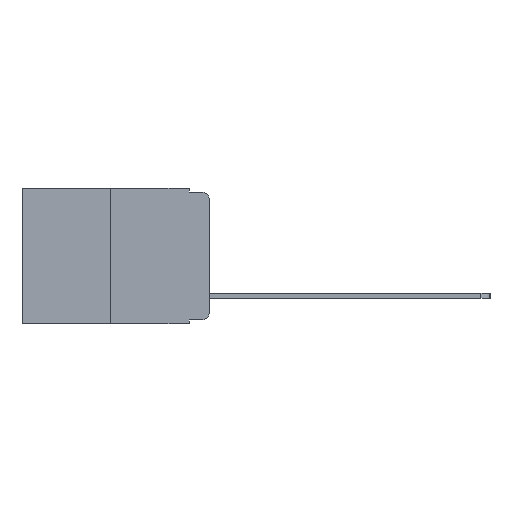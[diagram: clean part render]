
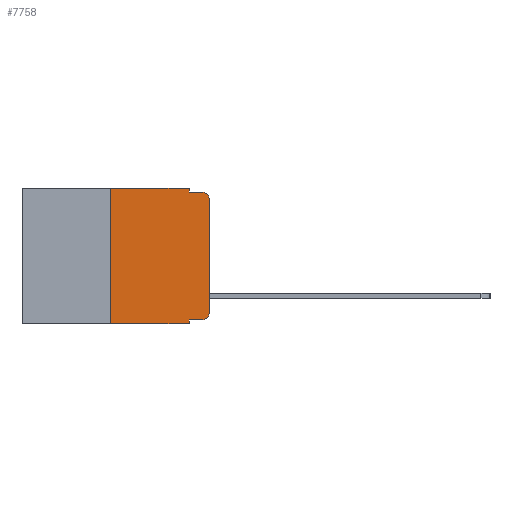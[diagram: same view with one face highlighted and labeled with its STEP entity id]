
A CAD part, left-side view. The second image highlights one B-rep face of the part: STEP entity #7758.
In plain terms, the highlighted planar face has unit normal (-1, 0, 0).
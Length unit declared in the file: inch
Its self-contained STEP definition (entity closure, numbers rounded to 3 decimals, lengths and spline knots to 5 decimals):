
#94 = CARTESIAN_POINT ( 'NONE',  ( 0., 0.051, 0. ) ) ;
#453 = VERTEX_POINT ( 'NONE', #15415 ) ;
#502 = VERTEX_POINT ( 'NONE', #5498 ) ;
#616 = VECTOR ( 'NONE', #14055, 39.37008 ) ;
#1423 = CARTESIAN_POINT ( 'NONE',  ( 0., 0.473, 0. ) ) ;
#1631 = DIRECTION ( 'NONE',  ( 0., -1., 0. ) ) ;
#1732 = LINE ( 'NONE', #10804, #14436 ) ;
#2265 = ORIENTED_EDGE ( 'NONE', *, *, #17275, .T. ) ;
#2407 = VERTEX_POINT ( 'NONE', #14971 ) ;
#2427 = VERTEX_POINT ( 'NONE', #5324 ) ;
#2765 = ORIENTED_EDGE ( 'NONE', *, *, #19211, .T. ) ;
#2782 = CARTESIAN_POINT ( 'NONE',  ( 0., 0.02, -0.03 ) ) ;
#2957 = DIRECTION ( 'NONE',  ( 1., 0., 0. ) ) ;
#3585 = LINE ( 'NONE', #4788, #7598 ) ;
#3799 = DIRECTION ( 'NONE',  ( 0., 0., -1. ) ) ;
#3984 = DIRECTION ( 'NONE',  ( 0., 0., 1. ) ) ;
#4356 = DIRECTION ( 'NONE',  ( 0., 0., -1. ) ) ;
#4765 = VERTEX_POINT ( 'NONE', #9627 ) ;
#4788 = CARTESIAN_POINT ( 'NONE',  ( 0., 0.051, -0.01 ) ) ;
#4835 = LINE ( 'NONE', #94, #616 ) ;
#4873 = LINE ( 'NONE', #11585, #12539 ) ;
#5050 = LINE ( 'NONE', #5389, #16146 ) ;
#5205 = EDGE_LOOP ( 'NONE', ( #2265, #2765, #18779, #7280, #11868, #8651, #16727, #13807, #17649, #14256 ) ) ;
#5324 = CARTESIAN_POINT ( 'NONE',  ( 0., 0., -0.313 ) ) ;
#5389 = CARTESIAN_POINT ( 'NONE',  ( 0., 0.473, -0.343 ) ) ;
#5498 = CARTESIAN_POINT ( 'NONE',  ( 0., 0.25, 0. ) ) ;
#5511 = EDGE_CURVE ( 'NONE', #453, #13199, #1732, .T. ) ;
#6650 = EDGE_CURVE ( 'NONE', #453, #4765, #13968, .T. ) ;
#7280 = ORIENTED_EDGE ( 'NONE', *, *, #8492, .F. ) ;
#7524 = EDGE_CURVE ( 'NONE', #13602, #502, #4873, .T. ) ;
#7598 = VECTOR ( 'NONE', #15340, 39.37008 ) ;
#7599 = CARTESIAN_POINT ( 'NONE',  ( 0., 0.02, -0.313 ) ) ;
#7758 = ADVANCED_FACE ( 'NONE', ( #16648 ), #8935, .F. ) ;
#8041 = LINE ( 'NONE', #17081, #11693 ) ;
#8492 = EDGE_CURVE ( 'NONE', #8644, #2407, #4835, .T. ) ;
#8644 = VERTEX_POINT ( 'NONE', #12850 ) ;
#8651 = ORIENTED_EDGE ( 'NONE', *, *, #7524, .F. ) ;
#8935 = PLANE ( 'NONE',  #12341 ) ;
#9086 = DIRECTION ( 'NONE',  ( 0., 0., -1. ) ) ;
#9311 = VECTOR ( 'NONE', #3799, 39.37008 ) ;
#9535 = EDGE_CURVE ( 'NONE', #2407, #9736, #3585, .T. ) ;
#9627 = CARTESIAN_POINT ( 'NONE',  ( 0., 0.051, -0.343 ) ) ;
#9736 = VERTEX_POINT ( 'NONE', #13211 ) ;
#9745 = AXIS2_PLACEMENT_3D ( 'NONE', #2782, #13508, #4356 ) ;
#10258 = VERTEX_POINT ( 'NONE', #19515 ) ;
#10804 = CARTESIAN_POINT ( 'NONE',  ( 0., 0.051, -0.333 ) ) ;
#11048 = CIRCLE ( 'NONE', #9745, 0.02 ) ;
#11113 = EDGE_CURVE ( 'NONE', #502, #8644, #13115, .T. ) ;
#11585 = CARTESIAN_POINT ( 'NONE',  ( 0., 0.25, 0. ) ) ;
#11693 = VECTOR ( 'NONE', #18552, 39.37008 ) ;
#11868 = ORIENTED_EDGE ( 'NONE', *, *, #11113, .F. ) ;
#11995 = CARTESIAN_POINT ( 'NONE',  ( 0., 0.02, -0.333 ) ) ;
#12129 = CARTESIAN_POINT ( 'NONE',  ( 0., 0.473, 0. ) ) ;
#12214 = DIRECTION ( 'NONE',  ( 0., -1., 0. ) ) ;
#12341 = AXIS2_PLACEMENT_3D ( 'NONE', #12129, #2957, #13673 ) ;
#12539 = VECTOR ( 'NONE', #3984, 39.37008 ) ;
#12850 = CARTESIAN_POINT ( 'NONE',  ( 0., 0.051, 0. ) ) ;
#12969 = CARTESIAN_POINT ( 'NONE',  ( 0., 0.051, 0. ) ) ;
#13115 = LINE ( 'NONE', #1423, #13592 ) ;
#13199 = VERTEX_POINT ( 'NONE', #11995 ) ;
#13211 = CARTESIAN_POINT ( 'NONE',  ( 0., 0.02, -0.01 ) ) ;
#13253 = AXIS2_PLACEMENT_3D ( 'NONE', #7599, #18105, #9086 ) ;
#13281 = EDGE_CURVE ( 'NONE', #13199, #2427, #18023, .T. ) ;
#13508 = DIRECTION ( 'NONE',  ( -1., 0., 0. ) ) ;
#13592 = VECTOR ( 'NONE', #12214, 39.37008 ) ;
#13602 = VERTEX_POINT ( 'NONE', #19166 ) ;
#13673 = DIRECTION ( 'NONE',  ( 0., 0., -1. ) ) ;
#13807 = ORIENTED_EDGE ( 'NONE', *, *, #6650, .F. ) ;
#13968 = LINE ( 'NONE', #12969, #9311 ) ;
#13977 = EDGE_CURVE ( 'NONE', #13602, #4765, #5050, .T. ) ;
#14055 = DIRECTION ( 'NONE',  ( 0., 0., -1. ) ) ;
#14256 = ORIENTED_EDGE ( 'NONE', *, *, #13281, .T. ) ;
#14436 = VECTOR ( 'NONE', #1631, 39.37008 ) ;
#14971 = CARTESIAN_POINT ( 'NONE',  ( 0., 0.051, -0.01 ) ) ;
#15340 = DIRECTION ( 'NONE',  ( 0., -1., 0. ) ) ;
#15415 = CARTESIAN_POINT ( 'NONE',  ( 0., 0.051, -0.333 ) ) ;
#15956 = DIRECTION ( 'NONE',  ( 0., -1., 0. ) ) ;
#16146 = VECTOR ( 'NONE', #15956, 39.37008 ) ;
#16648 = FACE_OUTER_BOUND ( 'NONE', #5205, .T. ) ;
#16727 = ORIENTED_EDGE ( 'NONE', *, *, #13977, .T. ) ;
#17081 = CARTESIAN_POINT ( 'NONE',  ( 0., 0., 0. ) ) ;
#17275 = EDGE_CURVE ( 'NONE', #2427, #10258, #8041, .T. ) ;
#17649 = ORIENTED_EDGE ( 'NONE', *, *, #5511, .T. ) ;
#18023 = CIRCLE ( 'NONE', #13253, 0.02 ) ;
#18105 = DIRECTION ( 'NONE',  ( -1., 0., 0. ) ) ;
#18552 = DIRECTION ( 'NONE',  ( 0., 0., 1. ) ) ;
#18779 = ORIENTED_EDGE ( 'NONE', *, *, #9535, .F. ) ;
#19166 = CARTESIAN_POINT ( 'NONE',  ( 0., 0.25, -0.343 ) ) ;
#19211 = EDGE_CURVE ( 'NONE', #10258, #9736, #11048, .T. ) ;
#19515 = CARTESIAN_POINT ( 'NONE',  ( 0., 0., -0.03 ) ) ;
